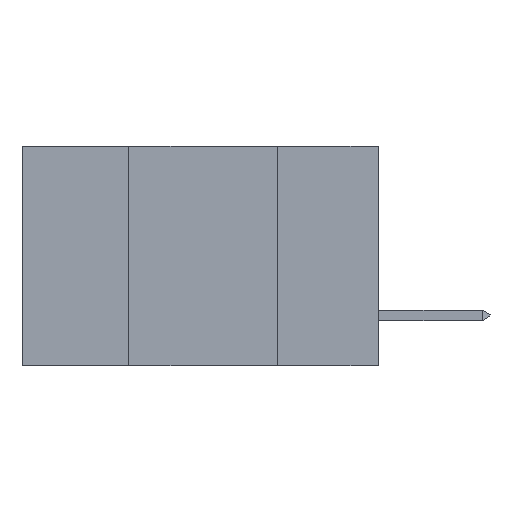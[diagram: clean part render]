
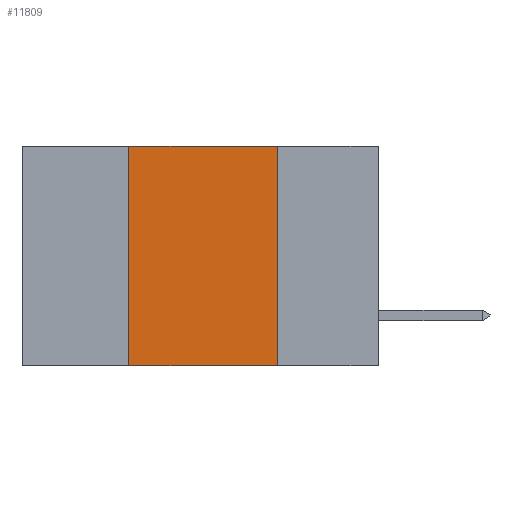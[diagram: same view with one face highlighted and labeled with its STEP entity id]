
A CAD part, left-side view. The second image highlights one B-rep face of the part: STEP entity #11809.
In plain terms, the highlighted planar face has unit normal (-1, 0, 0).
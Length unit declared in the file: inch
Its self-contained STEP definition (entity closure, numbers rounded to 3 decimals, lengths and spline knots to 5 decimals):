
#17 = VERTEX_POINT ( 'NONE', #8546 ) ;
#274 = EDGE_CURVE ( 'NONE', #6952, #17, #3443, .T. ) ;
#340 = EDGE_CURVE ( 'NONE', #6499, #3243, #1794, .T. ) ;
#398 = DIRECTION ( 'NONE',  ( 0., 0., -1. ) ) ;
#796 = ORIENTED_EDGE ( 'NONE', *, *, #11075, .F. ) ;
#1140 = DIRECTION ( 'NONE',  ( 0., -1., 0. ) ) ;
#1181 = CARTESIAN_POINT ( 'NONE',  ( 0., 0.6, -0.37 ) ) ;
#1396 = EDGE_CURVE ( 'NONE', #6499, #17, #2234, .T. ) ;
#1501 = ORIENTED_EDGE ( 'NONE', *, *, #1396, .T. ) ;
#1794 = LINE ( 'NONE', #6237, #7080 ) ;
#2157 = FACE_OUTER_BOUND ( 'NONE', #7299, .T. ) ;
#2168 = ORIENTED_EDGE ( 'NONE', *, *, #340, .F. ) ;
#2234 = LINE ( 'NONE', #1181, #8396 ) ;
#3243 = VERTEX_POINT ( 'NONE', #12350 ) ;
#3443 = LINE ( 'NONE', #9896, #4983 ) ;
#4983 = VECTOR ( 'NONE', #398, 39.37008 ) ;
#5975 = DIRECTION ( 'NONE',  ( 0., -1., 0. ) ) ;
#6237 = CARTESIAN_POINT ( 'NONE',  ( 0., 0.42, 0. ) ) ;
#6317 = DIRECTION ( 'NONE',  ( 0., 0., 1. ) ) ;
#6499 = VERTEX_POINT ( 'NONE', #11372 ) ;
#6699 = DIRECTION ( 'NONE',  ( 1., 0., 0. ) ) ;
#6952 = VERTEX_POINT ( 'NONE', #11563 ) ;
#7080 = VECTOR ( 'NONE', #6317, 39.37008 ) ;
#7299 = EDGE_LOOP ( 'NONE', ( #11357, #796, #2168, #1501 ) ) ;
#7437 = VECTOR ( 'NONE', #5975, 39.37008 ) ;
#8206 = AXIS2_PLACEMENT_3D ( 'NONE', #9680, #6699, #10675 ) ;
#8396 = VECTOR ( 'NONE', #1140, 39.37008 ) ;
#8546 = CARTESIAN_POINT ( 'NONE',  ( 0., 0.17, -0.37 ) ) ;
#8722 = PLANE ( 'NONE',  #8206 ) ;
#9680 = CARTESIAN_POINT ( 'NONE',  ( 0., 0.6, 0. ) ) ;
#9697 = LINE ( 'NONE', #11761, #7437 ) ;
#9896 = CARTESIAN_POINT ( 'NONE',  ( 0., 0.17, 0. ) ) ;
#10675 = DIRECTION ( 'NONE',  ( 0., 0., -1. ) ) ;
#11075 = EDGE_CURVE ( 'NONE', #3243, #6952, #9697, .T. ) ;
#11357 = ORIENTED_EDGE ( 'NONE', *, *, #274, .F. ) ;
#11372 = CARTESIAN_POINT ( 'NONE',  ( 0., 0.42, -0.37 ) ) ;
#11563 = CARTESIAN_POINT ( 'NONE',  ( 0., 0.17, 0. ) ) ;
#11761 = CARTESIAN_POINT ( 'NONE',  ( 0., 0.6, 0. ) ) ;
#11809 = ADVANCED_FACE ( 'NONE', ( #2157 ), #8722, .F. ) ;
#12350 = CARTESIAN_POINT ( 'NONE',  ( 0., 0.42, 0. ) ) ;
